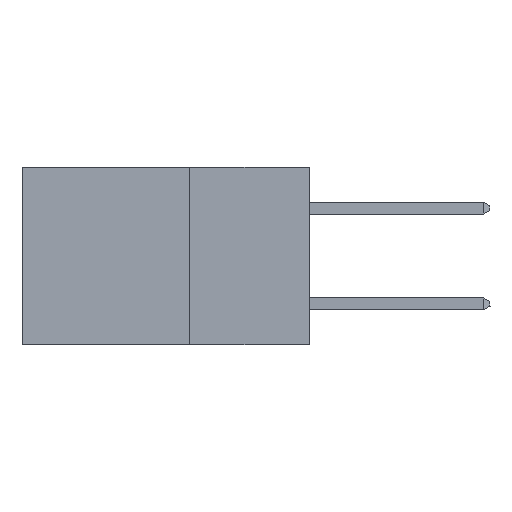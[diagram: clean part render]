
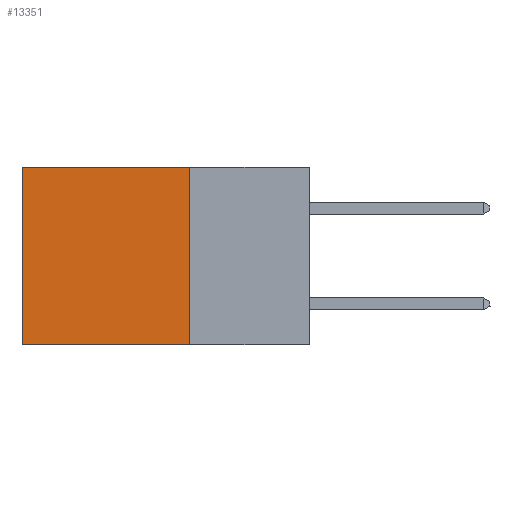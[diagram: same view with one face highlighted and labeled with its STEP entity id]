
A CAD part, left-side view. The second image highlights one B-rep face of the part: STEP entity #13351.
In plain terms, the highlighted planar face has unit normal (-1, 0, 0).
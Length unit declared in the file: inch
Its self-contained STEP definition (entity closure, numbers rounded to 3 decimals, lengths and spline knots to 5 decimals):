
#665 = DIRECTION ( 'NONE',  ( 0., 1., 0. ) ) ;
#1092 = CARTESIAN_POINT ( 'NONE',  ( 0.2875, 0.25, 0. ) ) ;
#1112 = DIRECTION ( 'NONE',  ( 0., 0., -1. ) ) ;
#1144 = CARTESIAN_POINT ( 'NONE',  ( 0.2875, 0.25, 0. ) ) ;
#1564 = VERTEX_POINT ( 'NONE', #2736 ) ;
#1841 = CARTESIAN_POINT ( 'NONE',  ( 0.2875, 0.6, 0. ) ) ;
#2736 = CARTESIAN_POINT ( 'NONE',  ( 0.2875, 0.25, 0. ) ) ;
#3807 = FACE_OUTER_BOUND ( 'NONE', #10094, .T. ) ;
#4513 = EDGE_CURVE ( 'NONE', #9138, #7096, #13021, .T. ) ;
#4551 = ORIENTED_EDGE ( 'NONE', *, *, #10239, .T. ) ;
#4738 = ORIENTED_EDGE ( 'NONE', *, *, #13810, .F. ) ;
#4826 = VECTOR ( 'NONE', #16103, 39.37008 ) ;
#4907 = AXIS2_PLACEMENT_3D ( 'NONE', #7953, #8123, #1112 ) ;
#6611 = ORIENTED_EDGE ( 'NONE', *, *, #7542, .T. ) ;
#7096 = VERTEX_POINT ( 'NONE', #7537 ) ;
#7237 = CARTESIAN_POINT ( 'NONE',  ( 0.2875, 0.25, -0.37 ) ) ;
#7340 = DIRECTION ( 'NONE',  ( 0., 0., -1. ) ) ;
#7537 = CARTESIAN_POINT ( 'NONE',  ( 0.2875, 0.6, -0.37 ) ) ;
#7542 = EDGE_CURVE ( 'NONE', #13651, #7096, #14183, .T. ) ;
#7953 = CARTESIAN_POINT ( 'NONE',  ( 0.2875, 0.25, 0. ) ) ;
#8103 = DIRECTION ( 'NONE',  ( 0., 0., -1. ) ) ;
#8123 = DIRECTION ( 'NONE',  ( 1., 0., 0. ) ) ;
#9138 = VERTEX_POINT ( 'NONE', #15429 ) ;
#9449 = LINE ( 'NONE', #1092, #15544 ) ;
#10094 = EDGE_LOOP ( 'NONE', ( #6611, #15181, #4738, #4551 ) ) ;
#10239 = EDGE_CURVE ( 'NONE', #1564, #13651, #14588, .T. ) ;
#10480 = CARTESIAN_POINT ( 'NONE',  ( 0.2875, 0.6, 0. ) ) ;
#10846 = PLANE ( 'NONE',  #4907 ) ;
#13021 = LINE ( 'NONE', #7237, #17108 ) ;
#13351 = ADVANCED_FACE ( 'NONE', ( #3807 ), #10846, .F. ) ;
#13651 = VERTEX_POINT ( 'NONE', #10480 ) ;
#13810 = EDGE_CURVE ( 'NONE', #1564, #9138, #9449, .T. ) ;
#14183 = LINE ( 'NONE', #1841, #15558 ) ;
#14588 = LINE ( 'NONE', #1144, #4826 ) ;
#15181 = ORIENTED_EDGE ( 'NONE', *, *, #4513, .F. ) ;
#15429 = CARTESIAN_POINT ( 'NONE',  ( 0.2875, 0.25, -0.37 ) ) ;
#15544 = VECTOR ( 'NONE', #8103, 39.37008 ) ;
#15558 = VECTOR ( 'NONE', #7340, 39.37008 ) ;
#16103 = DIRECTION ( 'NONE',  ( 0., 1., 0. ) ) ;
#17108 = VECTOR ( 'NONE', #665, 39.37008 ) ;
